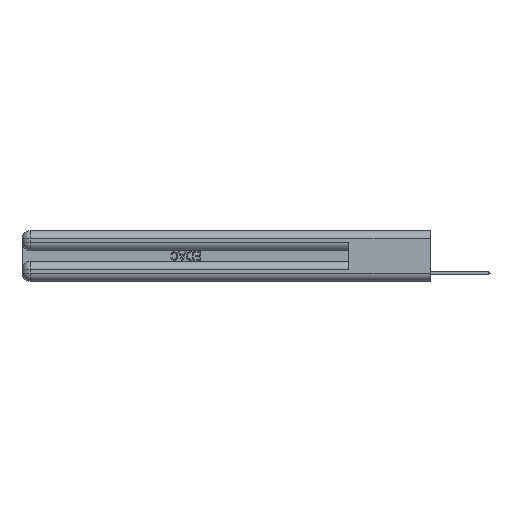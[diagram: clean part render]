
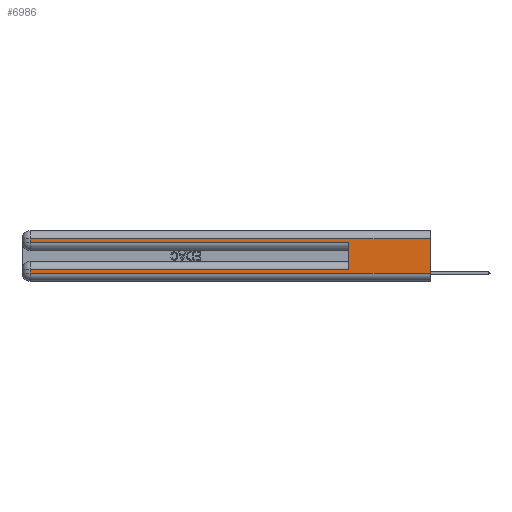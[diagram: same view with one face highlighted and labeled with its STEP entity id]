
A CAD part, left-side view. The second image highlights one B-rep face of the part: STEP entity #6986.
In plain terms, the highlighted planar face has unit normal (-1, 0, 0).
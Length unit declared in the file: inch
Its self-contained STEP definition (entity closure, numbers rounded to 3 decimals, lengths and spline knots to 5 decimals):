
#260 = LINE ( 'NONE', #10156, #28065 ) ;
#395 = VERTEX_POINT ( 'NONE', #3123 ) ;
#1168 = VECTOR ( 'NONE', #27749, 39.37008 ) ;
#1229 = AXIS2_PLACEMENT_3D ( 'NONE', #23814, #11894, #6603 ) ;
#1845 = EDGE_CURVE ( 'NONE', #31902, #10047, #2121, .T. ) ;
#2121 = LINE ( 'NONE', #24441, #19008 ) ;
#2442 = DIRECTION ( 'NONE',  ( 0., 1., 0. ) ) ;
#2881 = CARTESIAN_POINT ( 'NONE',  ( 0., 0.6, 0.085 ) ) ;
#2924 = EDGE_CURVE ( 'NONE', #395, #31187, #260, .T. ) ;
#3123 = CARTESIAN_POINT ( 'NONE',  ( 0., 2.94, 0.06 ) ) ;
#3716 = VERTEX_POINT ( 'NONE', #25658 ) ;
#5703 = CARTESIAN_POINT ( 'NONE',  ( 0., 0., 0.31 ) ) ;
#6251 = EDGE_LOOP ( 'NONE', ( #11393, #11269, #12095, #10757, #27586, #32165, #24217, #12170 ) ) ;
#6458 = EDGE_CURVE ( 'NONE', #14720, #25587, #25415, .T. ) ;
#6603 = DIRECTION ( 'NONE',  ( 0., 0., -1. ) ) ;
#6878 = VERTEX_POINT ( 'NONE', #2881 ) ;
#6986 = ADVANCED_FACE ( 'NONE', ( #16844 ), #9063, .F. ) ;
#7397 = EDGE_CURVE ( 'NONE', #3716, #395, #13522, .T. ) ;
#7696 = DIRECTION ( 'NONE',  ( 0., -1., 0. ) ) ;
#8019 = LINE ( 'NONE', #17638, #29729 ) ;
#8062 = VECTOR ( 'NONE', #2442, 39.37008 ) ;
#9063 = PLANE ( 'NONE',  #1229 ) ;
#10047 = VERTEX_POINT ( 'NONE', #24316 ) ;
#10156 = CARTESIAN_POINT ( 'NONE',  ( 0., 0., 0.06 ) ) ;
#10757 = ORIENTED_EDGE ( 'NONE', *, *, #1845, .T. ) ;
#11269 = ORIENTED_EDGE ( 'NONE', *, *, #6458, .T. ) ;
#11393 = ORIENTED_EDGE ( 'NONE', *, *, #12646, .F. ) ;
#11894 = DIRECTION ( 'NONE',  ( 1., 0., 0. ) ) ;
#12095 = ORIENTED_EDGE ( 'NONE', *, *, #32476, .T. ) ;
#12170 = ORIENTED_EDGE ( 'NONE', *, *, #2924, .T. ) ;
#12646 = EDGE_CURVE ( 'NONE', #14720, #31187, #8019, .T. ) ;
#13522 = LINE ( 'NONE', #29211, #31338 ) ;
#14720 = VERTEX_POINT ( 'NONE', #16106 ) ;
#15136 = VECTOR ( 'NONE', #31167, 39.37008 ) ;
#16106 = CARTESIAN_POINT ( 'NONE',  ( 0., 0., 0.31 ) ) ;
#16844 = FACE_OUTER_BOUND ( 'NONE', #6251, .T. ) ;
#17638 = CARTESIAN_POINT ( 'NONE',  ( 0., 0., 0.37 ) ) ;
#17966 = LINE ( 'NONE', #18130, #1168 ) ;
#18130 = CARTESIAN_POINT ( 'NONE',  ( 0., 2.94, 0.37 ) ) ;
#18942 = DIRECTION ( 'NONE',  ( 0., 0., -1. ) ) ;
#18948 = EDGE_CURVE ( 'NONE', #6878, #3716, #26585, .T. ) ;
#19008 = VECTOR ( 'NONE', #32359, 39.37008 ) ;
#21248 = CARTESIAN_POINT ( 'NONE',  ( 0., 0.6, 0.145 ) ) ;
#21905 = CARTESIAN_POINT ( 'NONE',  ( 0., 2.94, 0.31 ) ) ;
#23814 = CARTESIAN_POINT ( 'NONE',  ( 0., 0., 0.37 ) ) ;
#24217 = ORIENTED_EDGE ( 'NONE', *, *, #7397, .T. ) ;
#24316 = CARTESIAN_POINT ( 'NONE',  ( 0., 0.6, 0.285 ) ) ;
#24441 = CARTESIAN_POINT ( 'NONE',  ( 0., 0., 0.285 ) ) ;
#24784 = CARTESIAN_POINT ( 'NONE',  ( 0., 0., 0.06 ) ) ;
#25415 = LINE ( 'NONE', #5703, #8062 ) ;
#25587 = VERTEX_POINT ( 'NONE', #21905 ) ;
#25658 = CARTESIAN_POINT ( 'NONE',  ( 0., 2.94, 0.085 ) ) ;
#26585 = LINE ( 'NONE', #29394, #27517 ) ;
#26751 = DIRECTION ( 'NONE',  ( 0., 1., 0. ) ) ;
#26920 = EDGE_CURVE ( 'NONE', #6878, #10047, #31332, .T. ) ;
#27517 = VECTOR ( 'NONE', #26751, 39.37008 ) ;
#27586 = ORIENTED_EDGE ( 'NONE', *, *, #26920, .F. ) ;
#27749 = DIRECTION ( 'NONE',  ( 0., 0., -1. ) ) ;
#28065 = VECTOR ( 'NONE', #7696, 39.37008 ) ;
#28340 = CARTESIAN_POINT ( 'NONE',  ( 0., 2.94, 0.285 ) ) ;
#29211 = CARTESIAN_POINT ( 'NONE',  ( 0., 2.94, 0.37 ) ) ;
#29394 = CARTESIAN_POINT ( 'NONE',  ( 0., 0., 0.085 ) ) ;
#29729 = VECTOR ( 'NONE', #30206, 39.37008 ) ;
#30206 = DIRECTION ( 'NONE',  ( 0., 0., -1. ) ) ;
#31167 = DIRECTION ( 'NONE',  ( 0., 0., 1. ) ) ;
#31187 = VERTEX_POINT ( 'NONE', #24784 ) ;
#31332 = LINE ( 'NONE', #21248, #15136 ) ;
#31338 = VECTOR ( 'NONE', #18942, 39.37008 ) ;
#31902 = VERTEX_POINT ( 'NONE', #28340 ) ;
#32165 = ORIENTED_EDGE ( 'NONE', *, *, #18948, .T. ) ;
#32359 = DIRECTION ( 'NONE',  ( 0., -1., 0. ) ) ;
#32476 = EDGE_CURVE ( 'NONE', #25587, #31902, #17966, .T. ) ;
